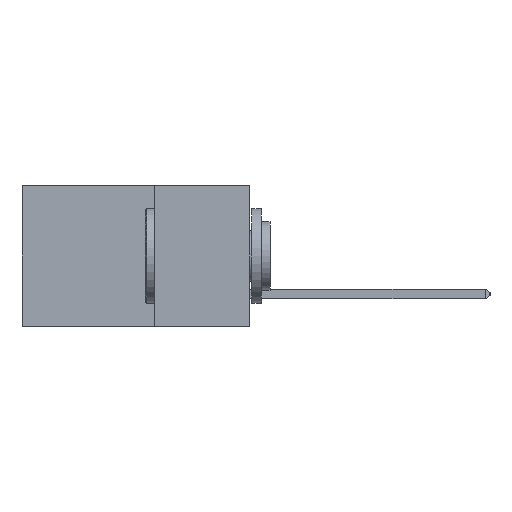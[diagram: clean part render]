
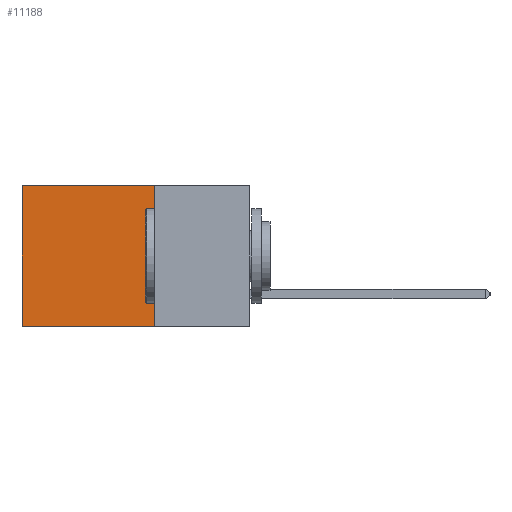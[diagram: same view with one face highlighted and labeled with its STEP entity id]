
A CAD part, left-side view. The second image highlights one B-rep face of the part: STEP entity #11188.
In plain terms, the highlighted planar face has unit normal (-1, 0, 0).
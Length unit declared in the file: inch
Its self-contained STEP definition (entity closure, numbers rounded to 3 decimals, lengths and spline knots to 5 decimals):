
#156 = VECTOR ( 'NONE', #5249, 39.37008 ) ;
#500 = EDGE_CURVE ( 'NONE', #21540, #6740, #10289, .T. ) ;
#977 = PLANE ( 'NONE',  #29704 ) ;
#1456 = ORIENTED_EDGE ( 'NONE', *, *, #31304, .F. ) ;
#3481 = DIRECTION ( 'NONE',  ( 0., 0., -1. ) ) ;
#3699 = VECTOR ( 'NONE', #9219, 39.37008 ) ;
#4748 = CARTESIAN_POINT ( 'NONE',  ( 0.2875, 0.25, 0. ) ) ;
#5249 = DIRECTION ( 'NONE',  ( 0., 1., 0. ) ) ;
#5628 = LINE ( 'NONE', #23430, #24722 ) ;
#5981 = LINE ( 'NONE', #17658, #156 ) ;
#6740 = VERTEX_POINT ( 'NONE', #31186 ) ;
#7646 = CARTESIAN_POINT ( 'NONE',  ( 0.2875, 0.25, -0.37 ) ) ;
#8231 = CARTESIAN_POINT ( 'NONE',  ( 0.2875, 0.25, 0. ) ) ;
#9219 = DIRECTION ( 'NONE',  ( 0., 1., 0. ) ) ;
#10289 = LINE ( 'NONE', #26650, #3699 ) ;
#10727 = DIRECTION ( 'NONE',  ( 0., 0., -1. ) ) ;
#10989 = LINE ( 'NONE', #8231, #16069 ) ;
#11006 = DIRECTION ( 'NONE',  ( 0., 0., -1. ) ) ;
#11188 = ADVANCED_FACE ( 'NONE', ( #32096 ), #977, .F. ) ;
#11984 = ORIENTED_EDGE ( 'NONE', *, *, #21894, .T. ) ;
#12617 = ORIENTED_EDGE ( 'NONE', *, *, #23084, .F. ) ;
#15755 = CARTESIAN_POINT ( 'NONE',  ( 0.2875, 0.25, 0. ) ) ;
#16069 = VECTOR ( 'NONE', #10727, 39.37008 ) ;
#16243 = CARTESIAN_POINT ( 'NONE',  ( 0.2875, 0.6, -0.37 ) ) ;
#17658 = CARTESIAN_POINT ( 'NONE',  ( 0.2875, 0.25, -0.37 ) ) ;
#18361 = DIRECTION ( 'NONE',  ( 1., 0., 0. ) ) ;
#21540 = VERTEX_POINT ( 'NONE', #4748 ) ;
#21667 = VERTEX_POINT ( 'NONE', #7646 ) ;
#21894 = EDGE_CURVE ( 'NONE', #6740, #25702, #5628, .T. ) ;
#23084 = EDGE_CURVE ( 'NONE', #21540, #21667, #10989, .T. ) ;
#23430 = CARTESIAN_POINT ( 'NONE',  ( 0.2875, 0.6, 0. ) ) ;
#24676 = ORIENTED_EDGE ( 'NONE', *, *, #500, .T. ) ;
#24722 = VECTOR ( 'NONE', #11006, 39.37008 ) ;
#25702 = VERTEX_POINT ( 'NONE', #16243 ) ;
#26650 = CARTESIAN_POINT ( 'NONE',  ( 0.2875, 0.25, 0. ) ) ;
#29704 = AXIS2_PLACEMENT_3D ( 'NONE', #15755, #18361, #3481 ) ;
#31186 = CARTESIAN_POINT ( 'NONE',  ( 0.2875, 0.6, 0. ) ) ;
#31304 = EDGE_CURVE ( 'NONE', #21667, #25702, #5981, .T. ) ;
#31493 = EDGE_LOOP ( 'NONE', ( #11984, #1456, #12617, #24676 ) ) ;
#32096 = FACE_OUTER_BOUND ( 'NONE', #31493, .T. ) ;
